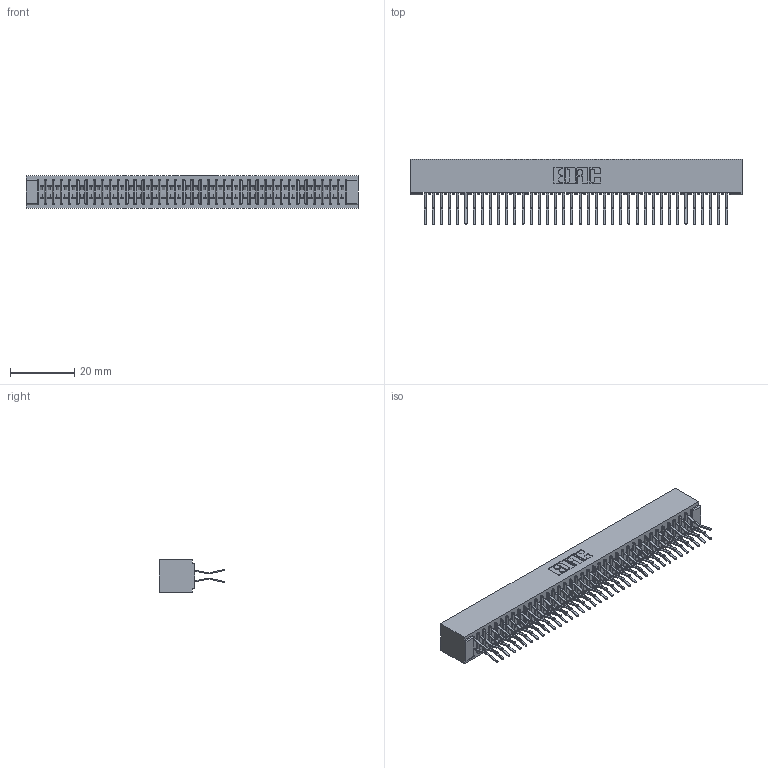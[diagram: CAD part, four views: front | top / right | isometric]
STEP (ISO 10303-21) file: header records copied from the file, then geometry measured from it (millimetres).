
FILE_DESCRIPTION (( 'STEP AP203' ), '1' );
FILE_NAME ('341-076-560-201.STEP', '2018-08-07T21:01:34', ( '' ), ( '' ), 'SwSTEP 2.0', 'SolidWorks 2016', '' );
FILE_SCHEMA (( 'CONFIG_CONTROL_DESIGN' ));
Length unit declared in the file: inch
Products named in the file (3): 341-292-001_341-292-160; 341-076-560-201; 341 Part_No Mounting Lugs
Assembly tree (77 placements, depth 2):
  341-076-560-201
    341 Part_No Mounting Lugs
    341-292-001_341-292-160  x76
Bounding box: 103.5 x 20.37 x 10.16 mm (x, y, z)
Volume: 7951.1 mm3; surface area: 15212.7 mm2
Topology: 77 solids, 77 shells, 5428 faces, 15758 edges, 10222 vertices
Faces by surface type: plane 3104, cylinder 2172, sphere 78, torus 74
Entity records: 46383 total; most frequent: CARTESIAN_POINT 7710, ORIENTED_EDGE 7660, DIRECTION 7488, EDGE_CURVE 3830, VECTOR 3088, LINE 3088, VERTEX_POINT 2422, AXIS2_PLACEMENT_3D 2200
